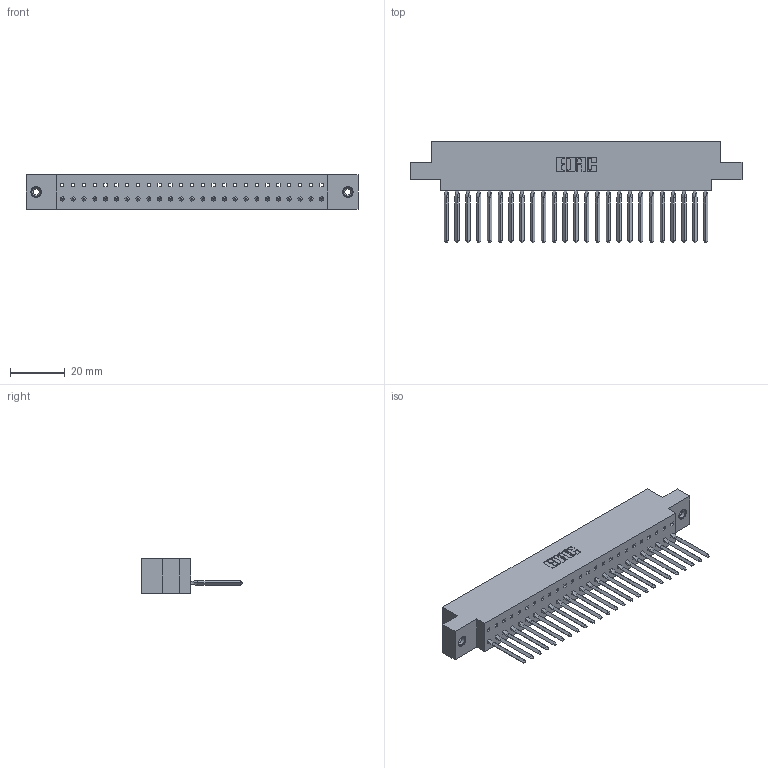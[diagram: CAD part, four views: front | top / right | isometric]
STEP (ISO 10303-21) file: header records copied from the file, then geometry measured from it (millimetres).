
FILE_DESCRIPTION (( 'STEP AP203' ), '1' );
FILE_NAME ('317-025-542-678.STEP', '2020-02-27T18:26:48', ( '' ), ( '' ), 'SwSTEP 2.0', 'SolidWorks 2016', '' );
FILE_SCHEMA (( 'CONFIG_CONTROL_DESIGN' ));
Length unit declared in the file: inch
Products named in the file (4): 317-025-542-678; 345-250-001_345-250-003-102; 317 Part_.156 Dia - TI; 317-290-003_542
Assembly tree (28 placements, depth 2):
  317-025-542-678
    317 Part_.156 Dia - TI
    317-290-003_542  x25
    345-250-001_345-250-003-102  x2
Bounding box: 121.77 x 37.34 x 12.7 mm (x, y, z)
Volume: 18351.3 mm3; surface area: 22028.7 mm2
Topology: 28 solids, 28 shells, 2037 faces, 5836 edges, 3766 vertices
Faces by surface type: plane 1690, cylinder 231, bspline 100, cone 12, torus 4
Entity records: 37912 total; most frequent: CARTESIAN_POINT 6947, ORIENTED_EDGE 6628, DIRECTION 5594, EDGE_CURVE 3314, VECTOR 3124, LINE 3124, VERTEX_POINT 2200, AXIS2_PLACEMENT_3D 1235
